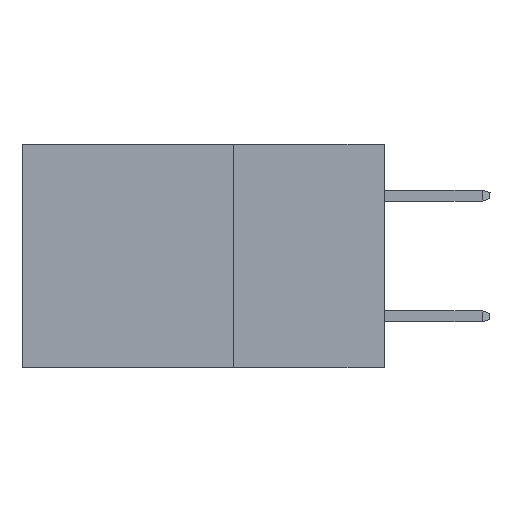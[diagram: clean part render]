
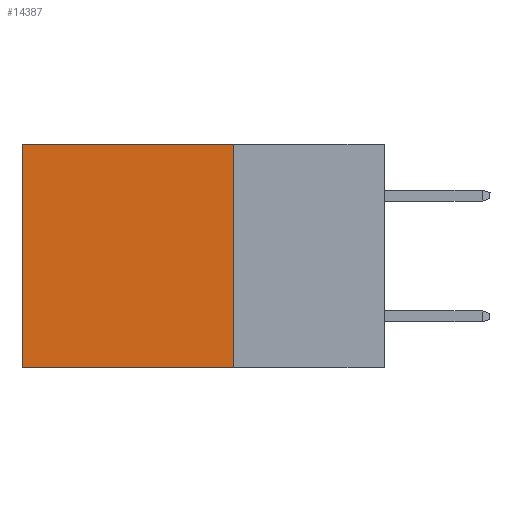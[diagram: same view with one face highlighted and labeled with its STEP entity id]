
A CAD part, left-side view. The second image highlights one B-rep face of the part: STEP entity #14387.
In plain terms, the highlighted planar face has unit normal (-1, 0, 0).
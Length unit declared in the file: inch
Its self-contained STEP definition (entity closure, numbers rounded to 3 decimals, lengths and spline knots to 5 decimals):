
#222 = DIRECTION ( 'NONE',  ( 0., 0., -1. ) ) ;
#297 = VERTEX_POINT ( 'NONE', #4284 ) ;
#963 = DIRECTION ( 'NONE',  ( 1., 0., 0. ) ) ;
#1475 = VERTEX_POINT ( 'NONE', #5137 ) ;
#1634 = CARTESIAN_POINT ( 'NONE',  ( 0.298, 0.25, -0.37 ) ) ;
#2680 = EDGE_CURVE ( 'NONE', #10653, #297, #12326, .T. ) ;
#3158 = LINE ( 'NONE', #1634, #13572 ) ;
#3413 = ORIENTED_EDGE ( 'NONE', *, *, #5602, .T. ) ;
#3414 = CARTESIAN_POINT ( 'NONE',  ( 0.298, 0.6, 0. ) ) ;
#4284 = CARTESIAN_POINT ( 'NONE',  ( 0.298, 0.6, -0.37 ) ) ;
#4513 = EDGE_LOOP ( 'NONE', ( #5415, #13186, #11472, #3413 ) ) ;
#4603 = CARTESIAN_POINT ( 'NONE',  ( 0.298, 0.25, 0. ) ) ;
#5137 = CARTESIAN_POINT ( 'NONE',  ( 0.298, 0.25, -0.37 ) ) ;
#5380 = DIRECTION ( 'NONE',  ( 0., 0., -1. ) ) ;
#5415 = ORIENTED_EDGE ( 'NONE', *, *, #2680, .T. ) ;
#5602 = EDGE_CURVE ( 'NONE', #13433, #10653, #12370, .T. ) ;
#5619 = DIRECTION ( 'NONE',  ( 0., 0., -1. ) ) ;
#6072 = DIRECTION ( 'NONE',  ( 0., 1., 0. ) ) ;
#6630 = EDGE_CURVE ( 'NONE', #1475, #297, #3158, .T. ) ;
#7227 = EDGE_CURVE ( 'NONE', #13433, #1475, #8118, .T. ) ;
#7691 = CARTESIAN_POINT ( 'NONE',  ( 0.298, 0.25, 0. ) ) ;
#7784 = CARTESIAN_POINT ( 'NONE',  ( 0.298, 0.25, 0. ) ) ;
#8118 = LINE ( 'NONE', #7784, #9850 ) ;
#9309 = VECTOR ( 'NONE', #222, 39.37008 ) ;
#9802 = CARTESIAN_POINT ( 'NONE',  ( 0.298, 0.6, 0. ) ) ;
#9850 = VECTOR ( 'NONE', #5619, 39.37008 ) ;
#9893 = PLANE ( 'NONE',  #12389 ) ;
#10653 = VERTEX_POINT ( 'NONE', #9802 ) ;
#11240 = FACE_OUTER_BOUND ( 'NONE', #4513, .T. ) ;
#11472 = ORIENTED_EDGE ( 'NONE', *, *, #7227, .F. ) ;
#11767 = DIRECTION ( 'NONE',  ( 0., 1., 0. ) ) ;
#12326 = LINE ( 'NONE', #3414, #9309 ) ;
#12370 = LINE ( 'NONE', #12731, #13955 ) ;
#12389 = AXIS2_PLACEMENT_3D ( 'NONE', #7691, #963, #5380 ) ;
#12731 = CARTESIAN_POINT ( 'NONE',  ( 0.298, 0.25, 0. ) ) ;
#13186 = ORIENTED_EDGE ( 'NONE', *, *, #6630, .F. ) ;
#13433 = VERTEX_POINT ( 'NONE', #4603 ) ;
#13572 = VECTOR ( 'NONE', #11767, 39.37008 ) ;
#13955 = VECTOR ( 'NONE', #6072, 39.37008 ) ;
#14387 = ADVANCED_FACE ( 'NONE', ( #11240 ), #9893, .F. ) ;
